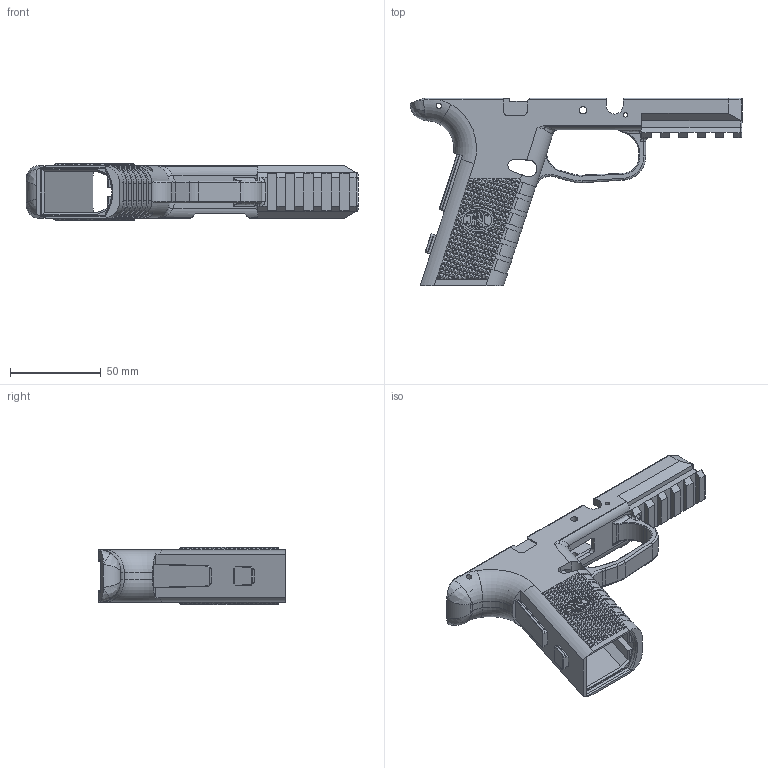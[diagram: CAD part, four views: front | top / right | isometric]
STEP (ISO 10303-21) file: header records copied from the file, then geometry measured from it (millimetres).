
FILE_DESCRIPTION(/* description */ (''),/* implementation_level */ '2;1');
FILE_NAME(/* name */ 'FNS-940_Texture_3 v2.step',/* time_stamp */ '2021-06-04T19:54:16-07:00',/* author */ (''),/* organization */ (''),/* preprocessor_version */ 'ST-DEVELOPER v18.1',/* originating_system */ 'Autodesk Translation Framework v10.9.0.1377',/* authorisation */ '');
FILE_SCHEMA (('AUTOMOTIVE_DESIGN { 1 0 10303 214 3 1 1 }'));
Products named in the file (5): FNS-940_Texture_3; Main Frame; Compact Size Grip; Standard Size Grip; Standard Size Grip (Stopgap)
Assembly tree (4 placements, depth 2):
  FNS-940_Texture_3
    Main Frame
    Compact Size Grip
    Standard Size Grip
    Standard Size Grip (Stopgap)
Bounding box: 183.1 x 103.6 x 31.54 mm (x, y, z)
Volume: 80992.2 mm3; surface area: 48089.7 mm2
Topology: 1 solids, 1 shells, 2955 faces, 6405 edges, 3457 vertices
Faces by surface type: plane 2629, cylinder 150, bspline 143, torus 27, cone 6
Full cylindrical faces by diameter (mm): 0.612 x2, 2.5 x2, 3 x2, 4.1 x2
Entity records: 91743 total; most frequent: CARTESIAN_POINT 29982, ORIENTED_EDGE 12806, DIRECTION 11966, EDGE_CURVE 6403, LINE 5542, VECTOR 5542, VERTEX_POINT 3457, AXIS2_PLACEMENT_3D 3212
